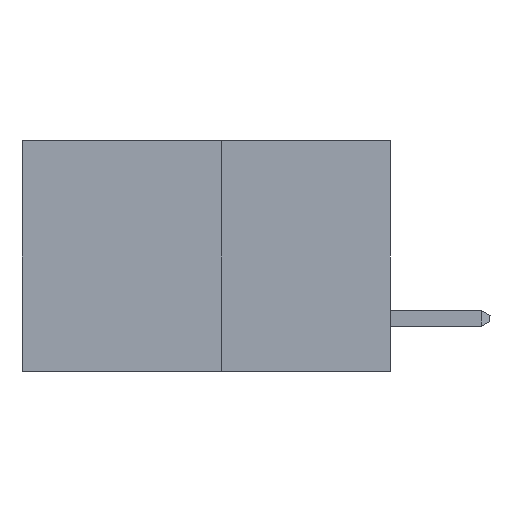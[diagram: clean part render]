
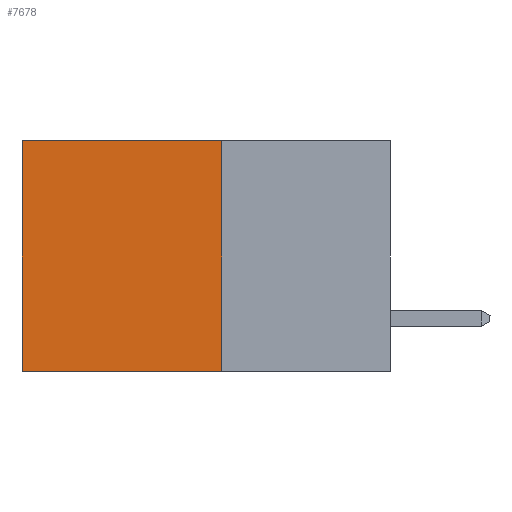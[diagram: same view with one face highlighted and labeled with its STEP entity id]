
A CAD part, left-side view. The second image highlights one B-rep face of the part: STEP entity #7678.
In plain terms, the highlighted planar face has unit normal (-1, 0, 0).
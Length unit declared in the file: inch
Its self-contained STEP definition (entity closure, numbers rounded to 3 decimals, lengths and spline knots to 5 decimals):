
#316 = CARTESIAN_POINT ( 'NONE',  ( 0.277, 0.59, -0.37 ) ) ;
#812 = AXIS2_PLACEMENT_3D ( 'NONE', #10476, #12733, #5896 ) ;
#1231 = EDGE_CURVE ( 'NONE', #10225, #6198, #8034, .T. ) ;
#1630 = VECTOR ( 'NONE', #12498, 39.37008 ) ;
#1758 = EDGE_CURVE ( 'NONE', #6198, #7081, #5320, .T. ) ;
#1965 = DIRECTION ( 'NONE',  ( 0., 1., 0. ) ) ;
#2222 = PLANE ( 'NONE',  #812 ) ;
#2336 = VECTOR ( 'NONE', #1965, 39.37008 ) ;
#2581 = DIRECTION ( 'NONE',  ( 0., 0., -1. ) ) ;
#2744 = CARTESIAN_POINT ( 'NONE',  ( 0.277, 0.27, -0.37 ) ) ;
#2890 = EDGE_CURVE ( 'NONE', #10225, #9499, #8116, .T. ) ;
#3462 = CARTESIAN_POINT ( 'NONE',  ( 0.277, 0.27, -0.37 ) ) ;
#3559 = EDGE_CURVE ( 'NONE', #9499, #7081, #11692, .T. ) ;
#4790 = CARTESIAN_POINT ( 'NONE',  ( 0.277, 0.59, 0. ) ) ;
#5082 = CARTESIAN_POINT ( 'NONE',  ( 0.277, 0.27, -0.37 ) ) ;
#5320 = LINE ( 'NONE', #316, #1630 ) ;
#5896 = DIRECTION ( 'NONE',  ( 0., 0., -1. ) ) ;
#6113 = CARTESIAN_POINT ( 'NONE',  ( 0.277, 0.59, -0.37 ) ) ;
#6191 = ORIENTED_EDGE ( 'NONE', *, *, #1758, .T. ) ;
#6198 = VERTEX_POINT ( 'NONE', #4790 ) ;
#7081 = VERTEX_POINT ( 'NONE', #6113 ) ;
#7553 = CARTESIAN_POINT ( 'NONE',  ( 0.277, 0.27, 0. ) ) ;
#7678 = ADVANCED_FACE ( 'NONE', ( #8062 ), #2222, .F. ) ;
#7780 = ORIENTED_EDGE ( 'NONE', *, *, #2890, .F. ) ;
#8034 = LINE ( 'NONE', #11198, #13722 ) ;
#8062 = FACE_OUTER_BOUND ( 'NONE', #9971, .T. ) ;
#8116 = LINE ( 'NONE', #3462, #11205 ) ;
#9499 = VERTEX_POINT ( 'NONE', #2744 ) ;
#9971 = EDGE_LOOP ( 'NONE', ( #6191, #12308, #7780, #12412 ) ) ;
#10225 = VERTEX_POINT ( 'NONE', #7553 ) ;
#10476 = CARTESIAN_POINT ( 'NONE',  ( 0.277, 0.27, -0.37 ) ) ;
#11198 = CARTESIAN_POINT ( 'NONE',  ( 0.277, 0.27, 0. ) ) ;
#11205 = VECTOR ( 'NONE', #2581, 39.37008 ) ;
#11692 = LINE ( 'NONE', #5082, #2336 ) ;
#12308 = ORIENTED_EDGE ( 'NONE', *, *, #3559, .F. ) ;
#12412 = ORIENTED_EDGE ( 'NONE', *, *, #1231, .T. ) ;
#12498 = DIRECTION ( 'NONE',  ( 0., 0., -1. ) ) ;
#12733 = DIRECTION ( 'NONE',  ( 1., 0., 0. ) ) ;
#13722 = VECTOR ( 'NONE', #14213, 39.37008 ) ;
#14213 = DIRECTION ( 'NONE',  ( 0., 1., 0. ) ) ;
